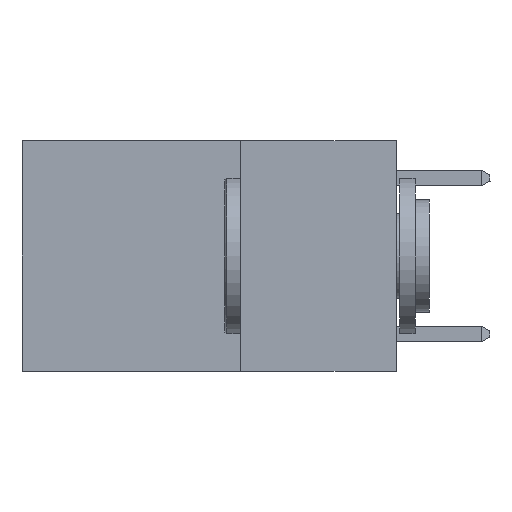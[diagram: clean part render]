
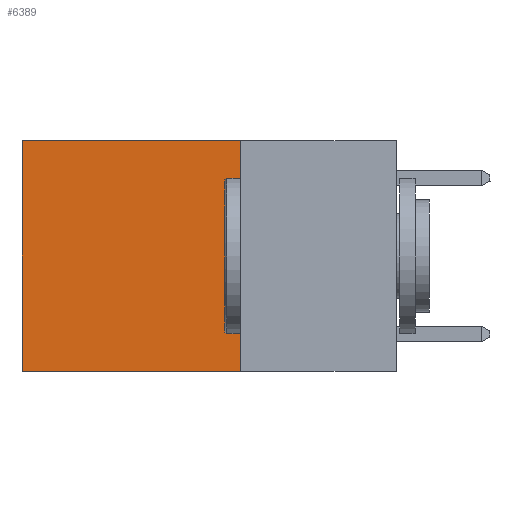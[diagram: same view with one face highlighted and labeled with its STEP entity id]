
A CAD part, left-side view. The second image highlights one B-rep face of the part: STEP entity #6389.
In plain terms, the highlighted planar face has unit normal (-1, 0, 0).
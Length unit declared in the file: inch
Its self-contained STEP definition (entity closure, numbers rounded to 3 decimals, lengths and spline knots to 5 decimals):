
#410 = VERTEX_POINT ( 'NONE', #19133 ) ;
#596 = EDGE_CURVE ( 'NONE', #6819, #410, #2337, .T. ) ;
#1246 = DIRECTION ( 'NONE',  ( 0., 0., -1. ) ) ;
#1636 = DIRECTION ( 'NONE',  ( 0., 0., -1. ) ) ;
#2337 = LINE ( 'NONE', #4439, #10496 ) ;
#2820 = LINE ( 'NONE', #14087, #18152 ) ;
#3239 = ORIENTED_EDGE ( 'NONE', *, *, #14211, .F. ) ;
#4439 = CARTESIAN_POINT ( 'NONE',  ( 0.2625, 0.6, 0. ) ) ;
#4822 = VECTOR ( 'NONE', #12923, 39.37008 ) ;
#5127 = CARTESIAN_POINT ( 'NONE',  ( 0.2625, 0.25, -0.37 ) ) ;
#5164 = DIRECTION ( 'NONE',  ( 0., 1., 0. ) ) ;
#6389 = ADVANCED_FACE ( 'NONE', ( #18972 ), #17517, .F. ) ;
#6819 = VERTEX_POINT ( 'NONE', #10732 ) ;
#6857 = CARTESIAN_POINT ( 'NONE',  ( 0.2625, 0.25, 0. ) ) ;
#6958 = CARTESIAN_POINT ( 'NONE',  ( 0.2625, 0.25, -0.37 ) ) ;
#7211 = DIRECTION ( 'NONE',  ( 0., 0., -1. ) ) ;
#7725 = ORIENTED_EDGE ( 'NONE', *, *, #14713, .F. ) ;
#9447 = VERTEX_POINT ( 'NONE', #6857 ) ;
#9898 = CARTESIAN_POINT ( 'NONE',  ( 0.2625, 0.25, 0. ) ) ;
#10383 = LINE ( 'NONE', #9898, #11093 ) ;
#10496 = VECTOR ( 'NONE', #1636, 39.37008 ) ;
#10732 = CARTESIAN_POINT ( 'NONE',  ( 0.2625, 0.6, 0. ) ) ;
#11093 = VECTOR ( 'NONE', #1246, 39.37008 ) ;
#12923 = DIRECTION ( 'NONE',  ( 0., 1., 0. ) ) ;
#13036 = EDGE_LOOP ( 'NONE', ( #13428, #7725, #3239, #17869 ) ) ;
#13385 = LINE ( 'NONE', #6958, #4822 ) ;
#13428 = ORIENTED_EDGE ( 'NONE', *, *, #596, .T. ) ;
#14087 = CARTESIAN_POINT ( 'NONE',  ( 0.2625, 0.25, 0. ) ) ;
#14211 = EDGE_CURVE ( 'NONE', #9447, #15350, #10383, .T. ) ;
#14687 = AXIS2_PLACEMENT_3D ( 'NONE', #17380, #19026, #7211 ) ;
#14713 = EDGE_CURVE ( 'NONE', #15350, #410, #13385, .T. ) ;
#15350 = VERTEX_POINT ( 'NONE', #5127 ) ;
#17380 = CARTESIAN_POINT ( 'NONE',  ( 0.2625, 0.25, 0. ) ) ;
#17517 = PLANE ( 'NONE',  #14687 ) ;
#17669 = EDGE_CURVE ( 'NONE', #9447, #6819, #2820, .T. ) ;
#17869 = ORIENTED_EDGE ( 'NONE', *, *, #17669, .T. ) ;
#18152 = VECTOR ( 'NONE', #5164, 39.37008 ) ;
#18972 = FACE_OUTER_BOUND ( 'NONE', #13036, .T. ) ;
#19026 = DIRECTION ( 'NONE',  ( 1., 0., 0. ) ) ;
#19133 = CARTESIAN_POINT ( 'NONE',  ( 0.2625, 0.6, -0.37 ) ) ;
